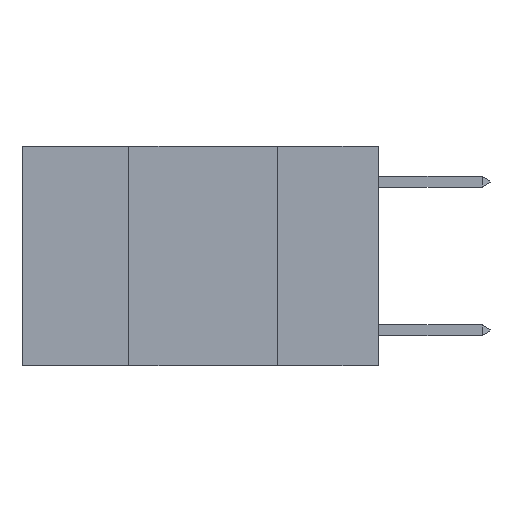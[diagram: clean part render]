
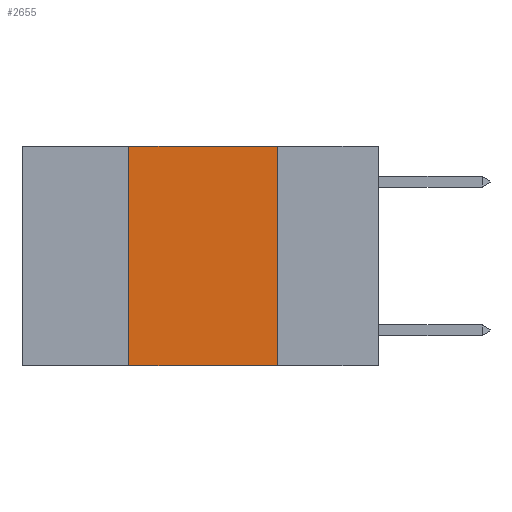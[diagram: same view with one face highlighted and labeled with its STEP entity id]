
A CAD part, left-side view. The second image highlights one B-rep face of the part: STEP entity #2655.
In plain terms, the highlighted planar face has unit normal (-1, 0, 0).
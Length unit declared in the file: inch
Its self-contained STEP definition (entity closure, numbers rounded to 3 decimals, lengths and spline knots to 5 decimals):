
#504 = ORIENTED_EDGE ( 'NONE', *, *, #23560, .F. ) ;
#1137 = DIRECTION ( 'NONE',  ( 0., 0., -1. ) ) ;
#1488 = LINE ( 'NONE', #21254, #19686 ) ;
#1851 = DIRECTION ( 'NONE',  ( 0., -1., 0. ) ) ;
#1877 = VECTOR ( 'NONE', #11077, 39.37008 ) ;
#2236 = DIRECTION ( 'NONE',  ( 0., 0., 1. ) ) ;
#2613 = LINE ( 'NONE', #30120, #1877 ) ;
#2655 = ADVANCED_FACE ( 'NONE', ( #26326 ), #10611, .F. ) ;
#2717 = ORIENTED_EDGE ( 'NONE', *, *, #13037, .F. ) ;
#2820 = CARTESIAN_POINT ( 'NONE',  ( 0., 0.17, 0. ) ) ;
#3323 = VECTOR ( 'NONE', #21848, 39.37008 ) ;
#3468 = CARTESIAN_POINT ( 'NONE',  ( 0., 0.17, 0. ) ) ;
#4074 = LINE ( 'NONE', #2820, #3323 ) ;
#5903 = VECTOR ( 'NONE', #1851, 39.37008 ) ;
#6531 = CARTESIAN_POINT ( 'NONE',  ( 0., 0.6, 0. ) ) ;
#7850 = VERTEX_POINT ( 'NONE', #25892 ) ;
#10057 = AXIS2_PLACEMENT_3D ( 'NONE', #29647, #15395, #1137 ) ;
#10611 = PLANE ( 'NONE',  #10057 ) ;
#10630 = CARTESIAN_POINT ( 'NONE',  ( 0., 0.17, -0.37 ) ) ;
#11077 = DIRECTION ( 'NONE',  ( 0., -1., 0. ) ) ;
#12255 = LINE ( 'NONE', #6531, #5903 ) ;
#13037 = EDGE_CURVE ( 'NONE', #14288, #7850, #1488, .T. ) ;
#13715 = EDGE_CURVE ( 'NONE', #7850, #16490, #12255, .T. ) ;
#13725 = ORIENTED_EDGE ( 'NONE', *, *, #23175, .T. ) ;
#14288 = VERTEX_POINT ( 'NONE', #17923 ) ;
#15395 = DIRECTION ( 'NONE',  ( 1., 0., 0. ) ) ;
#16490 = VERTEX_POINT ( 'NONE', #3468 ) ;
#17923 = CARTESIAN_POINT ( 'NONE',  ( 0., 0.42, -0.37 ) ) ;
#19686 = VECTOR ( 'NONE', #2236, 39.37008 ) ;
#21254 = CARTESIAN_POINT ( 'NONE',  ( 0., 0.42, 0. ) ) ;
#21848 = DIRECTION ( 'NONE',  ( 0., 0., -1. ) ) ;
#23175 = EDGE_CURVE ( 'NONE', #14288, #29200, #2613, .T. ) ;
#23560 = EDGE_CURVE ( 'NONE', #16490, #29200, #4074, .T. ) ;
#25892 = CARTESIAN_POINT ( 'NONE',  ( 0., 0.42, 0. ) ) ;
#26326 = FACE_OUTER_BOUND ( 'NONE', #30269, .T. ) ;
#28741 = ORIENTED_EDGE ( 'NONE', *, *, #13715, .F. ) ;
#29200 = VERTEX_POINT ( 'NONE', #10630 ) ;
#29647 = CARTESIAN_POINT ( 'NONE',  ( 0., 0.6, 0. ) ) ;
#30120 = CARTESIAN_POINT ( 'NONE',  ( 0., 0.6, -0.37 ) ) ;
#30269 = EDGE_LOOP ( 'NONE', ( #504, #28741, #2717, #13725 ) ) ;
